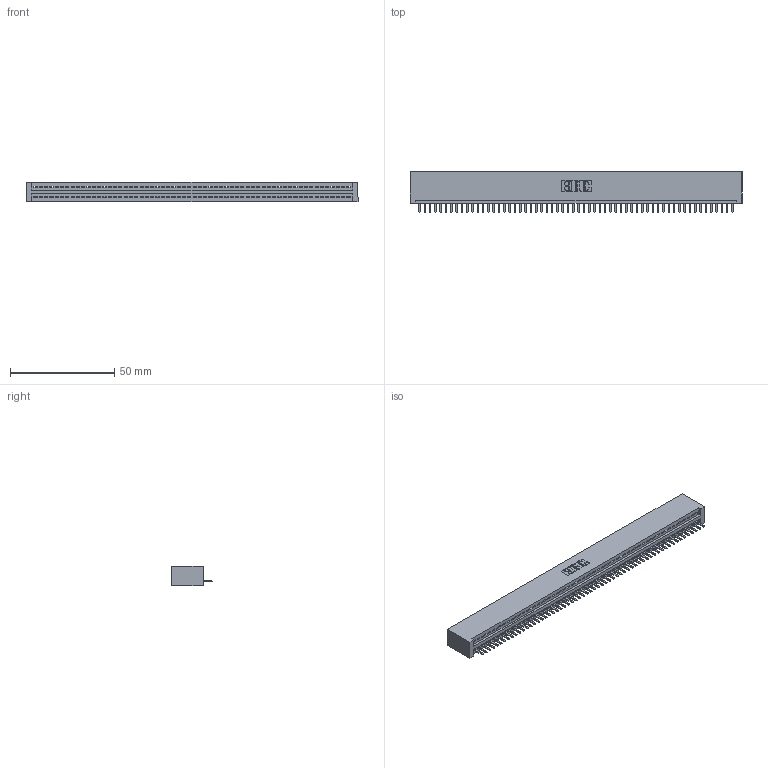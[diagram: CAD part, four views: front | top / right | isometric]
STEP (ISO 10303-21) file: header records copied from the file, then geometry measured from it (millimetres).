
FILE_DESCRIPTION (( 'STEP AP203' ), '1' );
FILE_NAME ('395-060-520-101.STEP', '2019-10-24T10:53:36', ( '' ), ( '' ), 'SwSTEP 2.0', 'SolidWorks 2016', '' );
FILE_SCHEMA (( 'CONFIG_CONTROL_DESIGN' ));
Length unit declared in the file: inch
Products named in the file (3): 345 Part_No Mounting Lugs; 395-060-520-101; 345-292-001_345-293-120
Assembly tree (61 placements, depth 2):
  395-060-520-101
    345 Part_No Mounting Lugs
    345-292-001_345-293-120  x60
Bounding box: 159 x 19.68 x 9.4 mm (x, y, z)
Volume: 15661.6 mm3; surface area: 20683 mm2
Topology: 61 solids, 61 shells, 3838 faces, 11357 edges, 7410 vertices
Faces by surface type: plane 2596, cylinder 1242
Entity records: 42571 total; most frequent: CARTESIAN_POINT 7392, ORIENTED_EDGE 7374, DIRECTION 6411, EDGE_CURVE 3687, LINE 3319, VECTOR 3319, VERTEX_POINT 2454, AXIS2_PLACEMENT_3D 1546
